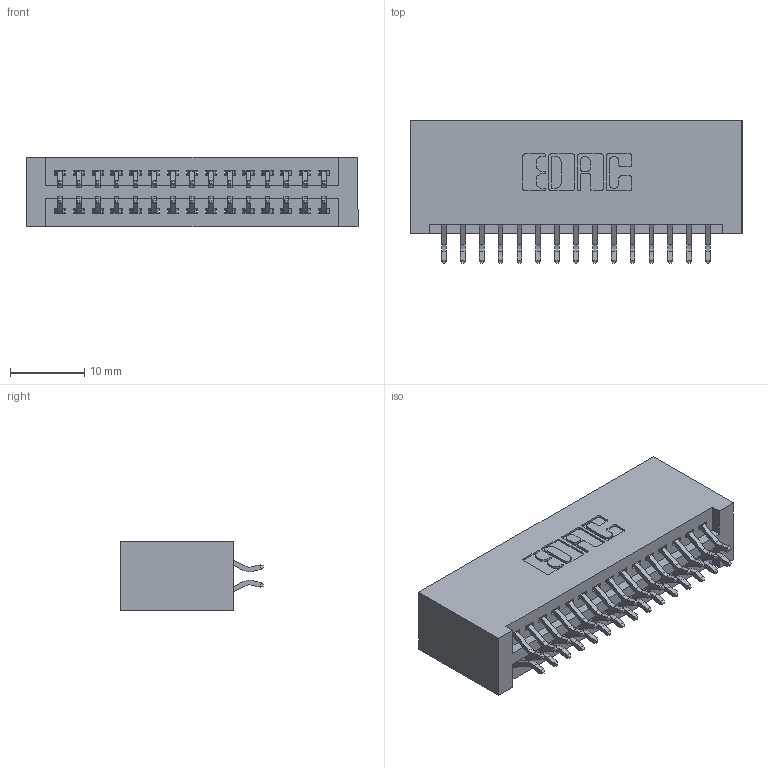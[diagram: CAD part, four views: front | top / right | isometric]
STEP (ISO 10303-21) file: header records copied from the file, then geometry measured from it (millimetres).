
FILE_DESCRIPTION (( 'STEP AP203' ), '1' );
FILE_NAME ('395-030-556-201.STEP', '2019-10-17T14:50:04', ( '' ), ( '' ), 'SwSTEP 2.0', 'SolidWorks 2016', '' );
FILE_SCHEMA (( 'CONFIG_CONTROL_DESIGN' ));
Length unit declared in the file: inch
Products named in the file (3): 345 Part_No Mounting Lugs; 345-292-001_556 Tail; 395-030-556-201
Assembly tree (31 placements, depth 2):
  395-030-556-201
    345 Part_No Mounting Lugs
    345-292-001_556 Tail  x30
Bounding box: 44.7 x 19.24 x 9.4 mm (x, y, z)
Volume: 4706.7 mm3; surface area: 6711.4 mm2
Topology: 31 solids, 31 shells, 1798 faces, 5327 edges, 3510 vertices
Faces by surface type: plane 1186, cylinder 612
Entity records: 15347 total; most frequent: CARTESIAN_POINT 2612, ORIENTED_EDGE 2534, DIRECTION 2319, EDGE_CURVE 1267, VECTOR 1075, LINE 1075, VERTEX_POINT 842, AXIS2_PLACEMENT_3D 622
